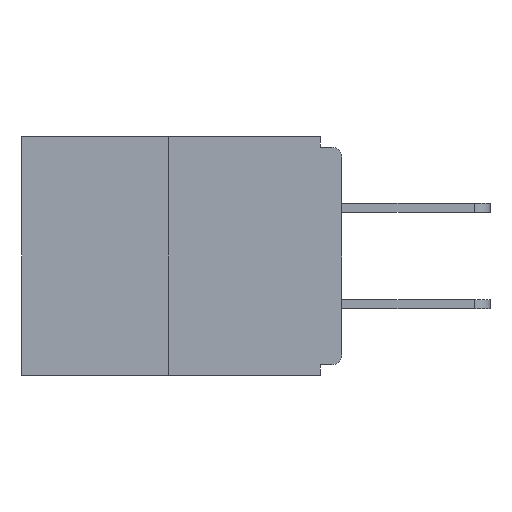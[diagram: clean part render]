
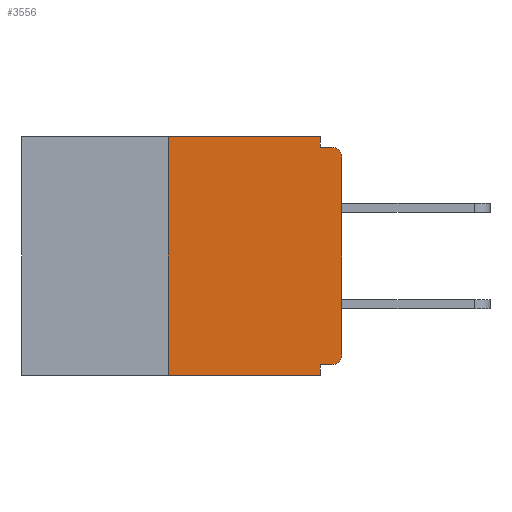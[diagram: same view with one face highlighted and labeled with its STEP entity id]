
A CAD part, left-side view. The second image highlights one B-rep face of the part: STEP entity #3556.
In plain terms, the highlighted planar face has unit normal (-1, 0, 0).
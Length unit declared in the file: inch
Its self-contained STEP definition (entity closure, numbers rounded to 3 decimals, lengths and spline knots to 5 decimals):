
#331 = CARTESIAN_POINT ( 'NONE',  ( 0., 0.015, -0.015 ) ) ;
#973 = EDGE_CURVE ( 'NONE', #11043, #9333, #18027, .T. ) ;
#1477 = EDGE_CURVE ( 'NONE', #20017, #21078, #10071, .T. ) ;
#1741 = DIRECTION ( 'NONE',  ( 0., 1., 0. ) ) ;
#2391 = DIRECTION ( 'NONE',  ( 0., 0., -1. ) ) ;
#2652 = LINE ( 'NONE', #4598, #19459 ) ;
#3395 = CARTESIAN_POINT ( 'NONE',  ( 0., 0., -0.03 ) ) ;
#3556 = ADVANCED_FACE ( 'NONE', ( #28170 ), #4437, .F. ) ;
#3786 = ORIENTED_EDGE ( 'NONE', *, *, #16148, .F. ) ;
#4174 = ORIENTED_EDGE ( 'NONE', *, *, #6815, .T. ) ;
#4333 = VECTOR ( 'NONE', #14806, 39.37008 ) ;
#4408 = DIRECTION ( 'NONE',  ( 0., 0., -1. ) ) ;
#4437 = PLANE ( 'NONE',  #22828 ) ;
#4598 = CARTESIAN_POINT ( 'NONE',  ( 0., 0.031, 0. ) ) ;
#4774 = CARTESIAN_POINT ( 'NONE',  ( 0., 0., 0. ) ) ;
#5266 = VERTEX_POINT ( 'NONE', #21086 ) ;
#5952 = EDGE_CURVE ( 'NONE', #21983, #5266, #24295, .T. ) ;
#6017 = EDGE_CURVE ( 'NONE', #22806, #11043, #2652, .T. ) ;
#6271 = CIRCLE ( 'NONE', #19920, 0.015 ) ;
#6437 = DIRECTION ( 'NONE',  ( 0., 0., 1. ) ) ;
#6815 = EDGE_CURVE ( 'NONE', #21078, #18573, #12651, .T. ) ;
#6874 = CARTESIAN_POINT ( 'NONE',  ( 0., 0.031, -0.343 ) ) ;
#6894 = EDGE_LOOP ( 'NONE', ( #12147, #27363, #9536, #9150, #3786, #13048, #4174, #12591, #27516, #15938 ) ) ;
#7636 = DIRECTION ( 'NONE',  ( 0., -1., 0. ) ) ;
#8194 = LINE ( 'NONE', #19027, #20849 ) ;
#8780 = VECTOR ( 'NONE', #7636, 39.37008 ) ;
#9034 = DIRECTION ( 'NONE',  ( 1., 0., 0. ) ) ;
#9077 = DIRECTION ( 'NONE',  ( 0., 0., -1. ) ) ;
#9150 = ORIENTED_EDGE ( 'NONE', *, *, #9763, .F. ) ;
#9333 = VERTEX_POINT ( 'NONE', #331 ) ;
#9536 = ORIENTED_EDGE ( 'NONE', *, *, #17995, .T. ) ;
#9763 = EDGE_CURVE ( 'NONE', #16916, #23853, #22531, .T. ) ;
#9772 = VECTOR ( 'NONE', #9077, 39.37008 ) ;
#10071 = CIRCLE ( 'NONE', #15210, 0.015 ) ;
#10115 = LINE ( 'NONE', #10414, #4333 ) ;
#10414 = CARTESIAN_POINT ( 'NONE',  ( 0., 0.46, 0. ) ) ;
#10775 = CARTESIAN_POINT ( 'NONE',  ( 0., 0.25, 0. ) ) ;
#11043 = VERTEX_POINT ( 'NONE', #19103 ) ;
#11538 = EDGE_CURVE ( 'NONE', #18573, #9333, #6271, .T. ) ;
#11746 = DIRECTION ( 'NONE',  ( 0., -1., 0. ) ) ;
#12062 = CARTESIAN_POINT ( 'NONE',  ( 0., 0.031, -0.343 ) ) ;
#12147 = ORIENTED_EDGE ( 'NONE', *, *, #27992, .F. ) ;
#12591 = ORIENTED_EDGE ( 'NONE', *, *, #11538, .T. ) ;
#12651 = LINE ( 'NONE', #4774, #23022 ) ;
#12927 = CARTESIAN_POINT ( 'NONE',  ( 0., 0., -0.015 ) ) ;
#12988 = DIRECTION ( 'NONE',  ( 0., 0., -1. ) ) ;
#13048 = ORIENTED_EDGE ( 'NONE', *, *, #1477, .T. ) ;
#13206 = CARTESIAN_POINT ( 'NONE',  ( 0., 0.46, 0. ) ) ;
#14806 = DIRECTION ( 'NONE',  ( 0., -1., 0. ) ) ;
#15210 = AXIS2_PLACEMENT_3D ( 'NONE', #23696, #17245, #12988 ) ;
#15684 = VECTOR ( 'NONE', #6437, 39.37008 ) ;
#15938 = ORIENTED_EDGE ( 'NONE', *, *, #6017, .F. ) ;
#16148 = EDGE_CURVE ( 'NONE', #20017, #16916, #8194, .T. ) ;
#16664 = DIRECTION ( 'NONE',  ( -1., 0., 0. ) ) ;
#16671 = CARTESIAN_POINT ( 'NONE',  ( 0., 0.015, -0.328 ) ) ;
#16755 = DIRECTION ( 'NONE',  ( 0., 0., -1. ) ) ;
#16916 = VERTEX_POINT ( 'NONE', #19893 ) ;
#17245 = DIRECTION ( 'NONE',  ( -1., 0., 0. ) ) ;
#17995 = EDGE_CURVE ( 'NONE', #21983, #23853, #27604, .T. ) ;
#18027 = LINE ( 'NONE', #12927, #8780 ) ;
#18573 = VERTEX_POINT ( 'NONE', #3395 ) ;
#19027 = CARTESIAN_POINT ( 'NONE',  ( 0., 0., -0.328 ) ) ;
#19103 = CARTESIAN_POINT ( 'NONE',  ( 0., 0.031, -0.015 ) ) ;
#19459 = VECTOR ( 'NONE', #4408, 39.37008 ) ;
#19893 = CARTESIAN_POINT ( 'NONE',  ( 0., 0.031, -0.328 ) ) ;
#19920 = AXIS2_PLACEMENT_3D ( 'NONE', #23033, #16664, #16755 ) ;
#20017 = VERTEX_POINT ( 'NONE', #16671 ) ;
#20482 = CARTESIAN_POINT ( 'NONE',  ( 0., 0.46, -0.343 ) ) ;
#20849 = VECTOR ( 'NONE', #1741, 39.37008 ) ;
#21078 = VERTEX_POINT ( 'NONE', #24905 ) ;
#21086 = CARTESIAN_POINT ( 'NONE',  ( 0., 0.25, 0. ) ) ;
#21426 = CARTESIAN_POINT ( 'NONE',  ( 0., 0.031, 0. ) ) ;
#21983 = VERTEX_POINT ( 'NONE', #22401 ) ;
#22401 = CARTESIAN_POINT ( 'NONE',  ( 0., 0.25, -0.343 ) ) ;
#22531 = LINE ( 'NONE', #6874, #9772 ) ;
#22806 = VERTEX_POINT ( 'NONE', #21426 ) ;
#22828 = AXIS2_PLACEMENT_3D ( 'NONE', #13206, #9034, #2391 ) ;
#23022 = VECTOR ( 'NONE', #24795, 39.37008 ) ;
#23033 = CARTESIAN_POINT ( 'NONE',  ( 0., 0.015, -0.03 ) ) ;
#23696 = CARTESIAN_POINT ( 'NONE',  ( 0., 0.015, -0.313 ) ) ;
#23853 = VERTEX_POINT ( 'NONE', #12062 ) ;
#24295 = LINE ( 'NONE', #10775, #15684 ) ;
#24795 = DIRECTION ( 'NONE',  ( 0., 0., 1. ) ) ;
#24905 = CARTESIAN_POINT ( 'NONE',  ( 0., 0., -0.313 ) ) ;
#26244 = VECTOR ( 'NONE', #11746, 39.37008 ) ;
#27363 = ORIENTED_EDGE ( 'NONE', *, *, #5952, .F. ) ;
#27516 = ORIENTED_EDGE ( 'NONE', *, *, #973, .F. ) ;
#27604 = LINE ( 'NONE', #20482, #26244 ) ;
#27992 = EDGE_CURVE ( 'NONE', #5266, #22806, #10115, .T. ) ;
#28170 = FACE_OUTER_BOUND ( 'NONE', #6894, .T. ) ;
